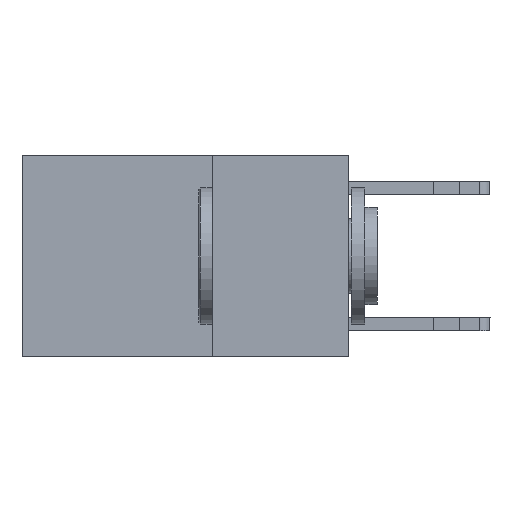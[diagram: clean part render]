
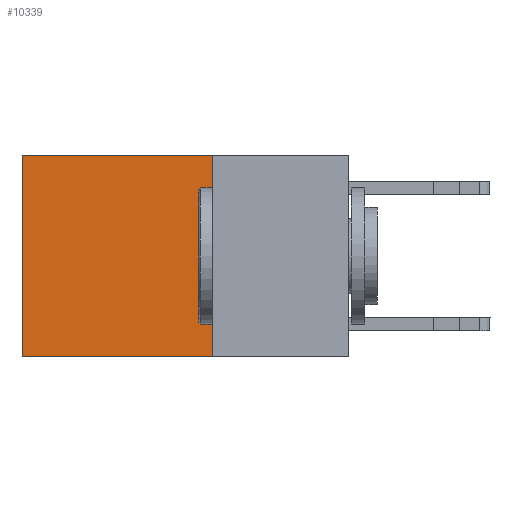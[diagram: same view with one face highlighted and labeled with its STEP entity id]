
A CAD part, left-side view. The second image highlights one B-rep face of the part: STEP entity #10339.
In plain terms, the highlighted planar face has unit normal (-1, 0, 0).
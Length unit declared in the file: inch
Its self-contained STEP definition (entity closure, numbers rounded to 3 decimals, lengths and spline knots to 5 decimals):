
#344 = DIRECTION ( 'NONE',  ( 0., 0., -1. ) ) ;
#481 = VECTOR ( 'NONE', #13299, 39.37008 ) ;
#724 = CARTESIAN_POINT ( 'NONE',  ( 0.2625, 0.25, 0. ) ) ;
#1466 = VERTEX_POINT ( 'NONE', #10507 ) ;
#1982 = DIRECTION ( 'NONE',  ( 1., 0., 0. ) ) ;
#2189 = ORIENTED_EDGE ( 'NONE', *, *, #7552, .F. ) ;
#3342 = EDGE_CURVE ( 'NONE', #1466, #3738, #12845, .T. ) ;
#3415 = CARTESIAN_POINT ( 'NONE',  ( 0.2625, 0.6, -0.37 ) ) ;
#3738 = VERTEX_POINT ( 'NONE', #3415 ) ;
#3872 = LINE ( 'NONE', #5939, #481 ) ;
#3899 = CARTESIAN_POINT ( 'NONE',  ( 0.2625, 0.25, 0. ) ) ;
#4303 = ORIENTED_EDGE ( 'NONE', *, *, #4612, .F. ) ;
#4612 = EDGE_CURVE ( 'NONE', #15153, #3738, #3872, .T. ) ;
#5148 = EDGE_LOOP ( 'NONE', ( #8740, #4303, #2189, #10382 ) ) ;
#5736 = VERTEX_POINT ( 'NONE', #6613 ) ;
#5939 = CARTESIAN_POINT ( 'NONE',  ( 0.2625, 0.25, -0.37 ) ) ;
#6613 = CARTESIAN_POINT ( 'NONE',  ( 0.2625, 0.25, 0. ) ) ;
#6624 = VECTOR ( 'NONE', #14913, 39.37008 ) ;
#7269 = CARTESIAN_POINT ( 'NONE',  ( 0.2625, 0.25, 0. ) ) ;
#7552 = EDGE_CURVE ( 'NONE', #5736, #15153, #13153, .T. ) ;
#7936 = CARTESIAN_POINT ( 'NONE',  ( 0.2625, 0.6, 0. ) ) ;
#8301 = PLANE ( 'NONE',  #12929 ) ;
#8740 = ORIENTED_EDGE ( 'NONE', *, *, #3342, .T. ) ;
#8852 = LINE ( 'NONE', #7269, #14845 ) ;
#8960 = CARTESIAN_POINT ( 'NONE',  ( 0.2625, 0.25, -0.37 ) ) ;
#10339 = ADVANCED_FACE ( 'NONE', ( #13790 ), #8301, .F. ) ;
#10382 = ORIENTED_EDGE ( 'NONE', *, *, #11193, .T. ) ;
#10507 = CARTESIAN_POINT ( 'NONE',  ( 0.2625, 0.6, 0. ) ) ;
#10794 = DIRECTION ( 'NONE',  ( 0., 0., -1. ) ) ;
#11193 = EDGE_CURVE ( 'NONE', #5736, #1466, #8852, .T. ) ;
#12486 = VECTOR ( 'NONE', #344, 39.37008 ) ;
#12845 = LINE ( 'NONE', #7936, #12486 ) ;
#12929 = AXIS2_PLACEMENT_3D ( 'NONE', #724, #1982, #10794 ) ;
#13153 = LINE ( 'NONE', #3899, #6624 ) ;
#13299 = DIRECTION ( 'NONE',  ( 0., 1., 0. ) ) ;
#13395 = DIRECTION ( 'NONE',  ( 0., 1., 0. ) ) ;
#13790 = FACE_OUTER_BOUND ( 'NONE', #5148, .T. ) ;
#14845 = VECTOR ( 'NONE', #13395, 39.37008 ) ;
#14913 = DIRECTION ( 'NONE',  ( 0., 0., -1. ) ) ;
#15153 = VERTEX_POINT ( 'NONE', #8960 ) ;
